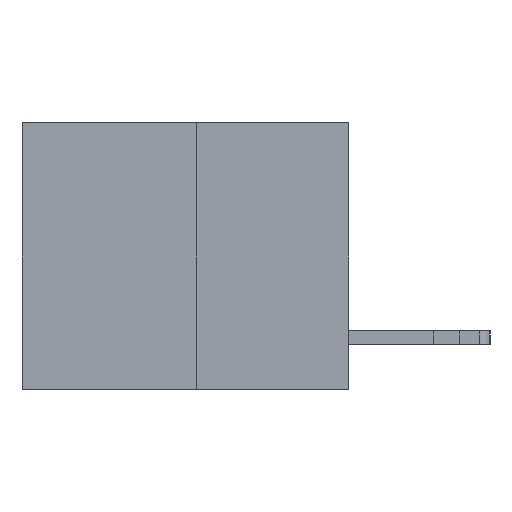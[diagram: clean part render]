
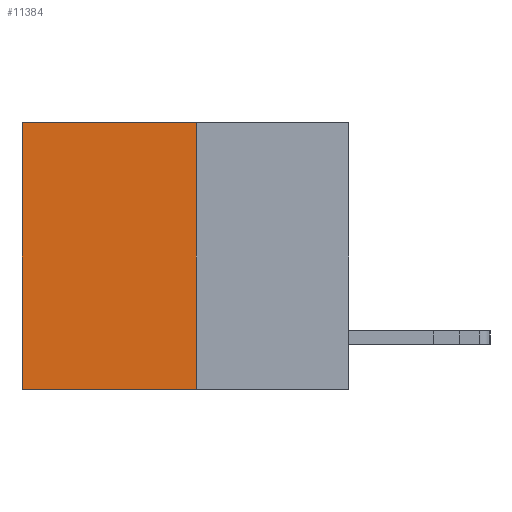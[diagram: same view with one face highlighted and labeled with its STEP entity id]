
A CAD part, left-side view. The second image highlights one B-rep face of the part: STEP entity #11384.
In plain terms, the highlighted planar face has unit normal (-1, 0, 0).
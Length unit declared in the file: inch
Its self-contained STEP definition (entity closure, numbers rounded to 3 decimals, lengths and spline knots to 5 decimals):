
#73 = VECTOR ( 'NONE', #3234, 39.37008 ) ;
#1337 = CARTESIAN_POINT ( 'NONE',  ( 0.3165, 0.28, 0. ) ) ;
#1538 = CARTESIAN_POINT ( 'NONE',  ( 0.3165, 0.28, -0.49 ) ) ;
#2843 = CARTESIAN_POINT ( 'NONE',  ( 0.3165, 0.28, 0. ) ) ;
#2883 = ORIENTED_EDGE ( 'NONE', *, *, #12870, .F. ) ;
#3105 = ORIENTED_EDGE ( 'NONE', *, *, #13993, .F. ) ;
#3112 = VECTOR ( 'NONE', #15895, 39.37008 ) ;
#3234 = DIRECTION ( 'NONE',  ( 0., 0., -1. ) ) ;
#3388 = VECTOR ( 'NONE', #6246, 39.37008 ) ;
#3665 = LINE ( 'NONE', #19444, #3112 ) ;
#6246 = DIRECTION ( 'NONE',  ( 0., 0., -1. ) ) ;
#6931 = EDGE_LOOP ( 'NONE', ( #20411, #2883, #3105, #14758 ) ) ;
#7235 = VERTEX_POINT ( 'NONE', #2843 ) ;
#7316 = CARTESIAN_POINT ( 'NONE',  ( 0.3165, 0.28, -0.49 ) ) ;
#8060 = CARTESIAN_POINT ( 'NONE',  ( 0.3165, 0.6, -0.49 ) ) ;
#8071 = LINE ( 'NONE', #1337, #11674 ) ;
#8142 = DIRECTION ( 'NONE',  ( 0., 1., 0. ) ) ;
#9185 = FACE_OUTER_BOUND ( 'NONE', #6931, .T. ) ;
#10347 = VERTEX_POINT ( 'NONE', #15969 ) ;
#11255 = EDGE_CURVE ( 'NONE', #7235, #20835, #8071, .T. ) ;
#11384 = ADVANCED_FACE ( 'NONE', ( #9185 ), #19256, .F. ) ;
#11674 = VECTOR ( 'NONE', #8142, 39.37008 ) ;
#12490 = EDGE_CURVE ( 'NONE', #20835, #10347, #21817, .T. ) ;
#12870 = EDGE_CURVE ( 'NONE', #21770, #10347, #3665, .T. ) ;
#13777 = DIRECTION ( 'NONE',  ( 0., 0., -1. ) ) ;
#13993 = EDGE_CURVE ( 'NONE', #7235, #21770, #17691, .T. ) ;
#14758 = ORIENTED_EDGE ( 'NONE', *, *, #11255, .T. ) ;
#15895 = DIRECTION ( 'NONE',  ( 0., 1., 0. ) ) ;
#15969 = CARTESIAN_POINT ( 'NONE',  ( 0.3165, 0.6, -0.49 ) ) ;
#17691 = LINE ( 'NONE', #20671, #73 ) ;
#19256 = PLANE ( 'NONE',  #20517 ) ;
#19444 = CARTESIAN_POINT ( 'NONE',  ( 0.3165, 0.28, -0.49 ) ) ;
#20411 = ORIENTED_EDGE ( 'NONE', *, *, #12490, .T. ) ;
#20517 = AXIS2_PLACEMENT_3D ( 'NONE', #1538, #22651, #13777 ) ;
#20671 = CARTESIAN_POINT ( 'NONE',  ( 0.3165, 0.28, -0.49 ) ) ;
#20835 = VERTEX_POINT ( 'NONE', #22031 ) ;
#21770 = VERTEX_POINT ( 'NONE', #7316 ) ;
#21817 = LINE ( 'NONE', #8060, #3388 ) ;
#22031 = CARTESIAN_POINT ( 'NONE',  ( 0.3165, 0.6, 0. ) ) ;
#22651 = DIRECTION ( 'NONE',  ( 1., 0., 0. ) ) ;
